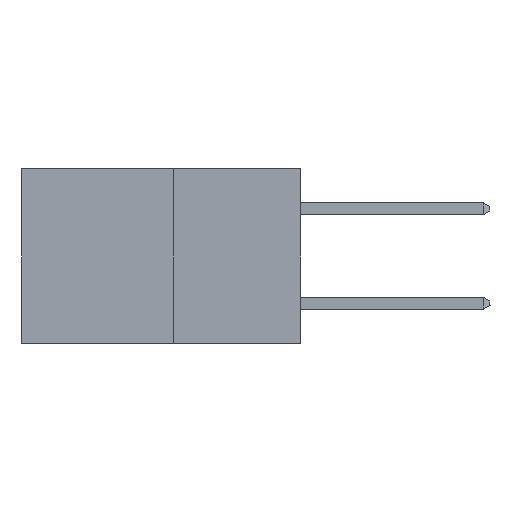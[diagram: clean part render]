
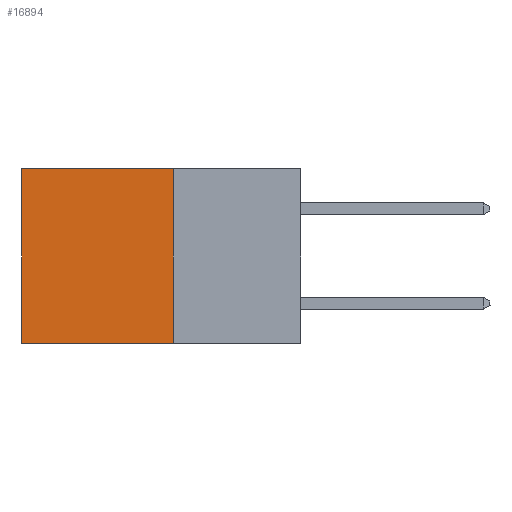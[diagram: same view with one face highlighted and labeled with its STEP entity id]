
A CAD part, left-side view. The second image highlights one B-rep face of the part: STEP entity #16894.
In plain terms, the highlighted planar face has unit normal (-1, 0, 0).
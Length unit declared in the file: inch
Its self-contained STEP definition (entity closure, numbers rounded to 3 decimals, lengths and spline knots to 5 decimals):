
#669 = CARTESIAN_POINT ( 'NONE',  ( 0.277, 0.59, 0. ) ) ;
#2847 = VECTOR ( 'NONE', #9991, 39.37008 ) ;
#3509 = FACE_OUTER_BOUND ( 'NONE', #10631, .T. ) ;
#3618 = VECTOR ( 'NONE', #24653, 39.37008 ) ;
#4152 = DIRECTION ( 'NONE',  ( 0., 0., -1. ) ) ;
#6742 = EDGE_CURVE ( 'NONE', #14721, #29152, #23316, .T. ) ;
#7019 = ORIENTED_EDGE ( 'NONE', *, *, #14695, .T. ) ;
#7350 = ORIENTED_EDGE ( 'NONE', *, *, #6742, .F. ) ;
#7425 = CARTESIAN_POINT ( 'NONE',  ( 0.277, 0.27, -0.37 ) ) ;
#7780 = CARTESIAN_POINT ( 'NONE',  ( 0.277, 0.27, 0. ) ) ;
#9130 = CARTESIAN_POINT ( 'NONE',  ( 0.277, 0.59, -0.37 ) ) ;
#9588 = LINE ( 'NONE', #9130, #3618 ) ;
#9991 = DIRECTION ( 'NONE',  ( 0., 0., -1. ) ) ;
#10044 = LINE ( 'NONE', #17270, #15292 ) ;
#10115 = CARTESIAN_POINT ( 'NONE',  ( 0.277, 0.27, 0. ) ) ;
#10631 = EDGE_LOOP ( 'NONE', ( #17686, #19985, #7350, #7019 ) ) ;
#14444 = EDGE_CURVE ( 'NONE', #28687, #30521, #9588, .T. ) ;
#14695 = EDGE_CURVE ( 'NONE', #14721, #28687, #22058, .T. ) ;
#14721 = VERTEX_POINT ( 'NONE', #7780 ) ;
#15292 = VECTOR ( 'NONE', #32798, 39.37008 ) ;
#16894 = ADVANCED_FACE ( 'NONE', ( #3509 ), #32339, .F. ) ;
#16912 = CARTESIAN_POINT ( 'NONE',  ( 0.277, 0.27, -0.37 ) ) ;
#17270 = CARTESIAN_POINT ( 'NONE',  ( 0.277, 0.27, -0.37 ) ) ;
#17686 = ORIENTED_EDGE ( 'NONE', *, *, #14444, .T. ) ;
#19479 = DIRECTION ( 'NONE',  ( 1., 0., 0. ) ) ;
#19985 = ORIENTED_EDGE ( 'NONE', *, *, #32430, .F. ) ;
#22058 = LINE ( 'NONE', #10115, #28115 ) ;
#23316 = LINE ( 'NONE', #7425, #2847 ) ;
#23791 = AXIS2_PLACEMENT_3D ( 'NONE', #16912, #19479, #4152 ) ;
#24653 = DIRECTION ( 'NONE',  ( 0., 0., -1. ) ) ;
#25524 = DIRECTION ( 'NONE',  ( 0., 1., 0. ) ) ;
#27818 = CARTESIAN_POINT ( 'NONE',  ( 0.277, 0.27, -0.37 ) ) ;
#28115 = VECTOR ( 'NONE', #25524, 39.37008 ) ;
#28687 = VERTEX_POINT ( 'NONE', #669 ) ;
#29152 = VERTEX_POINT ( 'NONE', #27818 ) ;
#30521 = VERTEX_POINT ( 'NONE', #32890 ) ;
#32339 = PLANE ( 'NONE',  #23791 ) ;
#32430 = EDGE_CURVE ( 'NONE', #29152, #30521, #10044, .T. ) ;
#32798 = DIRECTION ( 'NONE',  ( 0., 1., 0. ) ) ;
#32890 = CARTESIAN_POINT ( 'NONE',  ( 0.277, 0.59, -0.37 ) ) ;
